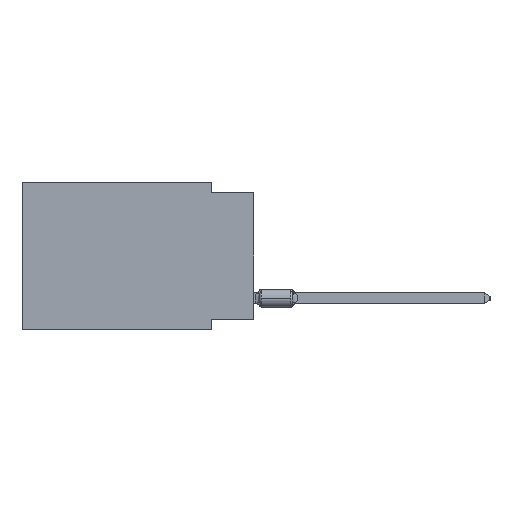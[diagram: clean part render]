
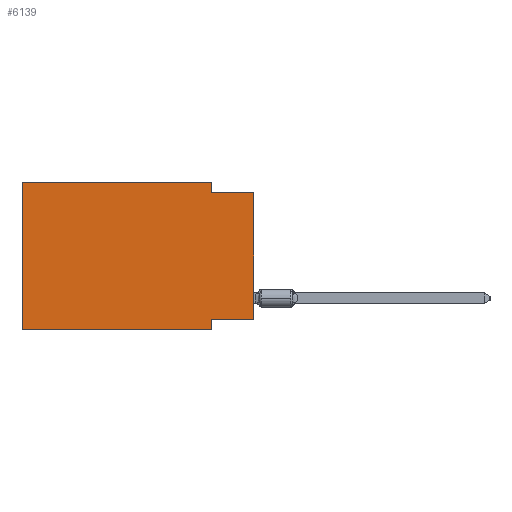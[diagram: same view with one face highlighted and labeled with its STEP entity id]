
A CAD part, left-side view. The second image highlights one B-rep face of the part: STEP entity #6139.
In plain terms, the highlighted planar face has unit normal (-1, 0, 0).
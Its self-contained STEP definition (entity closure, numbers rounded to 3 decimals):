
#65 = DIRECTION ( 'NONE',  ( 1., 0., 0. ) ) ;
#450 = EDGE_CURVE ( 'NONE', #38147, #46355, #22768, .T. ) ;
#1573 = CARTESIAN_POINT ( 'NONE',  ( 0., 2.54, 0. ) ) ;
#2848 = LINE ( 'NONE', #35600, #43109 ) ;
#4235 = LINE ( 'NONE', #18615, #40865 ) ;
#4912 = DIRECTION ( 'NONE',  ( 0., 1., 0. ) ) ;
#5134 = CARTESIAN_POINT ( 'NONE',  ( 0., 0., -8.255 ) ) ;
#5548 = CARTESIAN_POINT ( 'NONE',  ( 0., 13.97, 0. ) ) ;
#6139 = ADVANCED_FACE ( 'NONE', ( #31414 ), #35415, .F. ) ;
#6657 = CARTESIAN_POINT ( 'NONE',  ( 0., 13.97, -8.89 ) ) ;
#6798 = LINE ( 'NONE', #13630, #37348 ) ;
#7005 = EDGE_CURVE ( 'NONE', #7831, #46355, #6798, .T. ) ;
#7831 = VERTEX_POINT ( 'NONE', #6657 ) ;
#7949 = EDGE_CURVE ( 'NONE', #7831, #16699, #29736, .T. ) ;
#8260 = VERTEX_POINT ( 'NONE', #27810 ) ;
#9036 = VECTOR ( 'NONE', #43528, 1000. ) ;
#9473 = EDGE_CURVE ( 'NONE', #22168, #42984, #2848, .T. ) ;
#9631 = CARTESIAN_POINT ( 'NONE',  ( 0., 2.54, -8.89 ) ) ;
#10209 = DIRECTION ( 'NONE',  ( 0., 0., -1. ) ) ;
#10570 = ORIENTED_EDGE ( 'NONE', *, *, #9473, .F. ) ;
#11088 = ORIENTED_EDGE ( 'NONE', *, *, #17290, .F. ) ;
#12268 = VECTOR ( 'NONE', #34543, 1000. ) ;
#13630 = CARTESIAN_POINT ( 'NONE',  ( 0., 13.97, -8.89 ) ) ;
#16699 = VERTEX_POINT ( 'NONE', #34297 ) ;
#16884 = LINE ( 'NONE', #20174, #12268 ) ;
#17290 = EDGE_CURVE ( 'NONE', #42984, #8260, #4235, .T. ) ;
#17867 = VERTEX_POINT ( 'NONE', #31007 ) ;
#18363 = ORIENTED_EDGE ( 'NONE', *, *, #450, .F. ) ;
#18393 = ORIENTED_EDGE ( 'NONE', *, *, #37824, .F. ) ;
#18615 = CARTESIAN_POINT ( 'NONE',  ( 0., 0., -0.635 ) ) ;
#18975 = ORIENTED_EDGE ( 'NONE', *, *, #7005, .T. ) ;
#20174 = CARTESIAN_POINT ( 'NONE',  ( 0., 0., 0. ) ) ;
#21169 = DIRECTION ( 'NONE',  ( 0., -1., 0. ) ) ;
#22168 = VERTEX_POINT ( 'NONE', #1573 ) ;
#22414 = DIRECTION ( 'NONE',  ( 0., 0., 1. ) ) ;
#22463 = CARTESIAN_POINT ( 'NONE',  ( 0., 2.54, -8.255 ) ) ;
#22535 = CARTESIAN_POINT ( 'NONE',  ( 0., 2.54, -8.89 ) ) ;
#22768 = LINE ( 'NONE', #22535, #9036 ) ;
#23015 = AXIS2_PLACEMENT_3D ( 'NONE', #45785, #65, #10209 ) ;
#25689 = VECTOR ( 'NONE', #33135, 1000. ) ;
#26473 = VECTOR ( 'NONE', #22414, 1000. ) ;
#27810 = CARTESIAN_POINT ( 'NONE',  ( 0., 0., -0.635 ) ) ;
#27938 = CARTESIAN_POINT ( 'NONE',  ( 0., 2.54, -0.635 ) ) ;
#28806 = CARTESIAN_POINT ( 'NONE',  ( 0., 13.97, 0. ) ) ;
#29736 = LINE ( 'NONE', #28806, #26473 ) ;
#31007 = CARTESIAN_POINT ( 'NONE',  ( 0., 0., -8.255 ) ) ;
#31414 = FACE_OUTER_BOUND ( 'NONE', #33110, .T. ) ;
#32615 = EDGE_CURVE ( 'NONE', #17867, #8260, #16884, .T. ) ;
#33110 = EDGE_LOOP ( 'NONE', ( #34755, #11088, #10570, #18393, #36018, #18975, #18363, #35124 ) ) ;
#33135 = DIRECTION ( 'NONE',  ( 0., -1., 0. ) ) ;
#33379 = LINE ( 'NONE', #5548, #25689 ) ;
#33654 = LINE ( 'NONE', #5134, #37972 ) ;
#34297 = CARTESIAN_POINT ( 'NONE',  ( 0., 13.97, 0. ) ) ;
#34543 = DIRECTION ( 'NONE',  ( 0., 0., 1. ) ) ;
#34755 = ORIENTED_EDGE ( 'NONE', *, *, #32615, .T. ) ;
#35124 = ORIENTED_EDGE ( 'NONE', *, *, #36246, .F. ) ;
#35415 = PLANE ( 'NONE',  #23015 ) ;
#35600 = CARTESIAN_POINT ( 'NONE',  ( 0., 2.54, 0. ) ) ;
#36018 = ORIENTED_EDGE ( 'NONE', *, *, #7949, .F. ) ;
#36246 = EDGE_CURVE ( 'NONE', #17867, #38147, #33654, .T. ) ;
#37348 = VECTOR ( 'NONE', #21169, 1000. ) ;
#37824 = EDGE_CURVE ( 'NONE', #16699, #22168, #33379, .T. ) ;
#37972 = VECTOR ( 'NONE', #4912, 1000. ) ;
#38147 = VERTEX_POINT ( 'NONE', #22463 ) ;
#39372 = DIRECTION ( 'NONE',  ( 0., 0., -1. ) ) ;
#40752 = DIRECTION ( 'NONE',  ( 0., -1., 0. ) ) ;
#40865 = VECTOR ( 'NONE', #40752, 1000. ) ;
#42984 = VERTEX_POINT ( 'NONE', #27938 ) ;
#43109 = VECTOR ( 'NONE', #39372, 1000. ) ;
#43528 = DIRECTION ( 'NONE',  ( 0., 0., -1. ) ) ;
#45785 = CARTESIAN_POINT ( 'NONE',  ( 0., 13.97, 0. ) ) ;
#46355 = VERTEX_POINT ( 'NONE', #9631 ) ;
